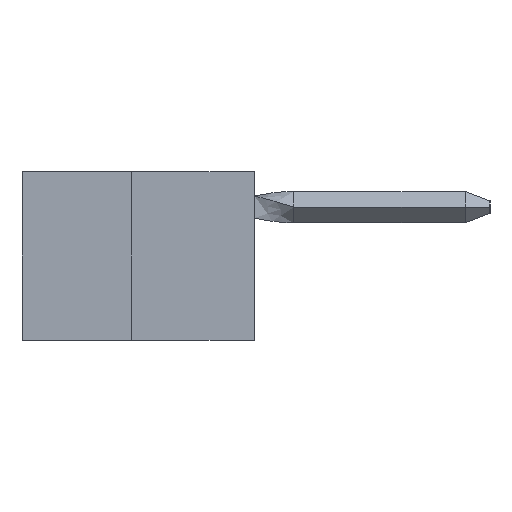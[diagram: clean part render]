
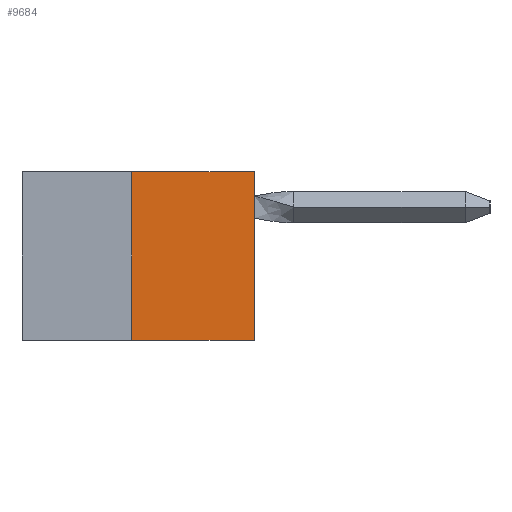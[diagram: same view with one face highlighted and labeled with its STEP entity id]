
A CAD part, left-side view. The second image highlights one B-rep face of the part: STEP entity #9684.
In plain terms, the highlighted planar face has unit normal (-1, 0, 0).
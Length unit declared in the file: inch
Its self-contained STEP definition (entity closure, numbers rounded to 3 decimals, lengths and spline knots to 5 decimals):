
#309 = DIRECTION ( 'NONE',  ( 0., 0., 1. ) ) ;
#426 = DIRECTION ( 'NONE',  ( 0., -1., 0. ) ) ;
#1004 = DIRECTION ( 'NONE',  ( 1., 0., 0. ) ) ;
#1057 = CARTESIAN_POINT ( 'NONE',  ( 0., 0.473, -0.343 ) ) ;
#1798 = CARTESIAN_POINT ( 'NONE',  ( 0., 0., 0. ) ) ;
#2111 = CARTESIAN_POINT ( 'NONE',  ( 0., 0.473, 0. ) ) ;
#2126 = ORIENTED_EDGE ( 'NONE', *, *, #7423, .F. ) ;
#2841 = EDGE_CURVE ( 'NONE', #11613, #19267, #4335, .T. ) ;
#2898 = VECTOR ( 'NONE', #426, 39.37008 ) ;
#3682 = ORIENTED_EDGE ( 'NONE', *, *, #2841, .T. ) ;
#3761 = EDGE_CURVE ( 'NONE', #19267, #20170, #21736, .T. ) ;
#4335 = LINE ( 'NONE', #1057, #14450 ) ;
#5177 = CARTESIAN_POINT ( 'NONE',  ( 0., 0.25, -0.343 ) ) ;
#7183 = ORIENTED_EDGE ( 'NONE', *, *, #7625, .F. ) ;
#7423 = EDGE_CURVE ( 'NONE', #8489, #20170, #13554, .T. ) ;
#7625 = EDGE_CURVE ( 'NONE', #11613, #8489, #12716, .T. ) ;
#8029 = CARTESIAN_POINT ( 'NONE',  ( 0., 0., 0. ) ) ;
#8489 = VERTEX_POINT ( 'NONE', #19725 ) ;
#9684 = ADVANCED_FACE ( 'NONE', ( #16988 ), #20117, .F. ) ;
#9930 = CARTESIAN_POINT ( 'NONE',  ( 0., 0., -0.343 ) ) ;
#11465 = DIRECTION ( 'NONE',  ( 0., -1., 0. ) ) ;
#11613 = VERTEX_POINT ( 'NONE', #5177 ) ;
#12716 = LINE ( 'NONE', #20800, #14358 ) ;
#13554 = LINE ( 'NONE', #2111, #2898 ) ;
#14358 = VECTOR ( 'NONE', #309, 39.37008 ) ;
#14450 = VECTOR ( 'NONE', #11465, 39.37008 ) ;
#16014 = ORIENTED_EDGE ( 'NONE', *, *, #3761, .T. ) ;
#16727 = DIRECTION ( 'NONE',  ( 0., 0., -1. ) ) ;
#16874 = CARTESIAN_POINT ( 'NONE',  ( 0., 0.473, 0. ) ) ;
#16988 = FACE_OUTER_BOUND ( 'NONE', #19909, .T. ) ;
#17143 = VECTOR ( 'NONE', #20112, 39.37008 ) ;
#17578 = AXIS2_PLACEMENT_3D ( 'NONE', #16874, #1004, #16727 ) ;
#19267 = VERTEX_POINT ( 'NONE', #9930 ) ;
#19725 = CARTESIAN_POINT ( 'NONE',  ( 0., 0.25, 0. ) ) ;
#19909 = EDGE_LOOP ( 'NONE', ( #2126, #7183, #3682, #16014 ) ) ;
#20112 = DIRECTION ( 'NONE',  ( 0., 0., 1. ) ) ;
#20117 = PLANE ( 'NONE',  #17578 ) ;
#20170 = VERTEX_POINT ( 'NONE', #1798 ) ;
#20800 = CARTESIAN_POINT ( 'NONE',  ( 0., 0.25, 0. ) ) ;
#21736 = LINE ( 'NONE', #8029, #17143 ) ;
